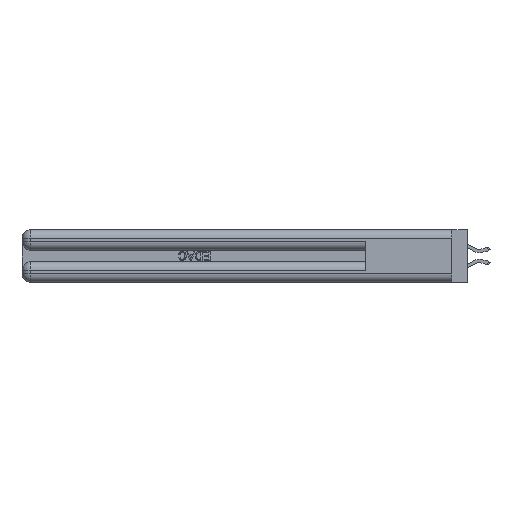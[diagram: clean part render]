
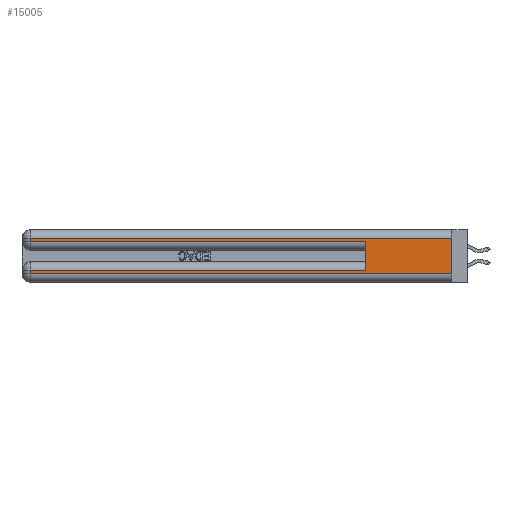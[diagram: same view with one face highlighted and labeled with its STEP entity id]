
A CAD part, left-side view. The second image highlights one B-rep face of the part: STEP entity #15005.
In plain terms, the highlighted planar face has unit normal (-1, 0, 0).
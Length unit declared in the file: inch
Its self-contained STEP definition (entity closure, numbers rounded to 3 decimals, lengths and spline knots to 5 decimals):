
#395 = CARTESIAN_POINT ( 'NONE',  ( 0., 0., 0.285 ) ) ;
#668 = ORIENTED_EDGE ( 'NONE', *, *, #1446, .T. ) ;
#1446 = EDGE_CURVE ( 'NONE', #40558, #11171, #9795, .T. ) ;
#1795 = LINE ( 'NONE', #11634, #26145 ) ;
#2205 = AXIS2_PLACEMENT_3D ( 'NONE', #20071, #23288, #4260 ) ;
#2228 = VERTEX_POINT ( 'NONE', #19326 ) ;
#3708 = VECTOR ( 'NONE', #14556, 39.37008 ) ;
#3912 = LINE ( 'NONE', #37819, #28234 ) ;
#4260 = DIRECTION ( 'NONE',  ( 0., 0., -1. ) ) ;
#5401 = DIRECTION ( 'NONE',  ( 0., 0., -1. ) ) ;
#5893 = EDGE_CURVE ( 'NONE', #12497, #40558, #39780, .T. ) ;
#7774 = ORIENTED_EDGE ( 'NONE', *, *, #8793, .F. ) ;
#8201 = CARTESIAN_POINT ( 'NONE',  ( 0., 2.94, 0.37 ) ) ;
#8793 = EDGE_CURVE ( 'NONE', #14598, #38057, #1795, .T. ) ;
#9157 = CARTESIAN_POINT ( 'NONE',  ( 0., 2.94, 0.37 ) ) ;
#9795 = LINE ( 'NONE', #9157, #26656 ) ;
#10900 = EDGE_CURVE ( 'NONE', #12497, #2228, #3912, .T. ) ;
#11171 = VERTEX_POINT ( 'NONE', #36982 ) ;
#11634 = CARTESIAN_POINT ( 'NONE',  ( 0., 0., 0.37 ) ) ;
#12425 = CARTESIAN_POINT ( 'NONE',  ( 0., 2.94, 0.285 ) ) ;
#12497 = VERTEX_POINT ( 'NONE', #40362 ) ;
#13572 = LINE ( 'NONE', #22555, #20991 ) ;
#14208 = CARTESIAN_POINT ( 'NONE',  ( 0., 0., 0.085 ) ) ;
#14469 = VECTOR ( 'NONE', #26975, 39.37008 ) ;
#14556 = DIRECTION ( 'NONE',  ( 0., 0., -1. ) ) ;
#14598 = VERTEX_POINT ( 'NONE', #27749 ) ;
#15005 = ADVANCED_FACE ( 'NONE', ( #35872 ), #16903, .F. ) ;
#16903 = PLANE ( 'NONE',  #2205 ) ;
#17977 = EDGE_CURVE ( 'NONE', #24259, #2228, #20549, .T. ) ;
#18352 = DIRECTION ( 'NONE',  ( 0., -1., 0. ) ) ;
#18661 = EDGE_CURVE ( 'NONE', #14598, #34922, #13572, .T. ) ;
#18688 = ORIENTED_EDGE ( 'NONE', *, *, #10900, .F. ) ;
#18946 = ORIENTED_EDGE ( 'NONE', *, *, #17977, .T. ) ;
#19326 = CARTESIAN_POINT ( 'NONE',  ( 0., 0.6, 0.285 ) ) ;
#19595 = ORIENTED_EDGE ( 'NONE', *, *, #5893, .T. ) ;
#20071 = CARTESIAN_POINT ( 'NONE',  ( 0., 0., 0.37 ) ) ;
#20549 = LINE ( 'NONE', #395, #36438 ) ;
#20567 = LINE ( 'NONE', #8201, #3708 ) ;
#20991 = VECTOR ( 'NONE', #35153, 39.37008 ) ;
#21575 = ORIENTED_EDGE ( 'NONE', *, *, #24907, .T. ) ;
#22369 = LINE ( 'NONE', #24741, #37241 ) ;
#22555 = CARTESIAN_POINT ( 'NONE',  ( 0., 0., 0.31 ) ) ;
#23288 = DIRECTION ( 'NONE',  ( 1., 0., 0. ) ) ;
#24259 = VERTEX_POINT ( 'NONE', #12425 ) ;
#24741 = CARTESIAN_POINT ( 'NONE',  ( 0., 0., 0.06 ) ) ;
#24907 = EDGE_CURVE ( 'NONE', #11171, #38057, #22369, .T. ) ;
#25015 = CARTESIAN_POINT ( 'NONE',  ( 0., 2.94, 0.31 ) ) ;
#26145 = VECTOR ( 'NONE', #5401, 39.37008 ) ;
#26656 = VECTOR ( 'NONE', #31339, 39.37008 ) ;
#26923 = CARTESIAN_POINT ( 'NONE',  ( 0., 2.94, 0.085 ) ) ;
#26975 = DIRECTION ( 'NONE',  ( 0., 1., 0. ) ) ;
#27749 = CARTESIAN_POINT ( 'NONE',  ( 0., 0., 0.31 ) ) ;
#28234 = VECTOR ( 'NONE', #41004, 39.37008 ) ;
#28579 = EDGE_CURVE ( 'NONE', #34922, #24259, #20567, .T. ) ;
#29433 = ORIENTED_EDGE ( 'NONE', *, *, #18661, .T. ) ;
#31339 = DIRECTION ( 'NONE',  ( 0., 0., -1. ) ) ;
#32172 = DIRECTION ( 'NONE',  ( 0., -1., 0. ) ) ;
#32675 = EDGE_LOOP ( 'NONE', ( #7774, #29433, #40051, #18946, #18688, #19595, #668, #21575 ) ) ;
#33608 = CARTESIAN_POINT ( 'NONE',  ( 0., 0., 0.06 ) ) ;
#34922 = VERTEX_POINT ( 'NONE', #25015 ) ;
#35153 = DIRECTION ( 'NONE',  ( 0., 1., 0. ) ) ;
#35872 = FACE_OUTER_BOUND ( 'NONE', #32675, .T. ) ;
#36438 = VECTOR ( 'NONE', #32172, 39.37008 ) ;
#36982 = CARTESIAN_POINT ( 'NONE',  ( 0., 2.94, 0.06 ) ) ;
#37241 = VECTOR ( 'NONE', #18352, 39.37008 ) ;
#37819 = CARTESIAN_POINT ( 'NONE',  ( 0., 0.6, 0.145 ) ) ;
#38057 = VERTEX_POINT ( 'NONE', #33608 ) ;
#39780 = LINE ( 'NONE', #14208, #14469 ) ;
#40051 = ORIENTED_EDGE ( 'NONE', *, *, #28579, .T. ) ;
#40362 = CARTESIAN_POINT ( 'NONE',  ( 0., 0.6, 0.085 ) ) ;
#40558 = VERTEX_POINT ( 'NONE', #26923 ) ;
#41004 = DIRECTION ( 'NONE',  ( 0., 0., 1. ) ) ;
